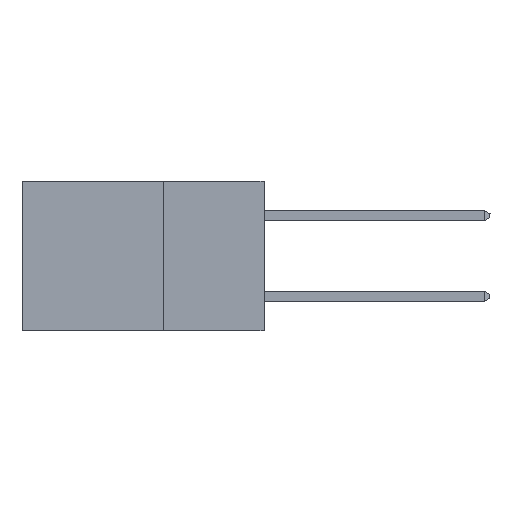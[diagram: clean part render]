
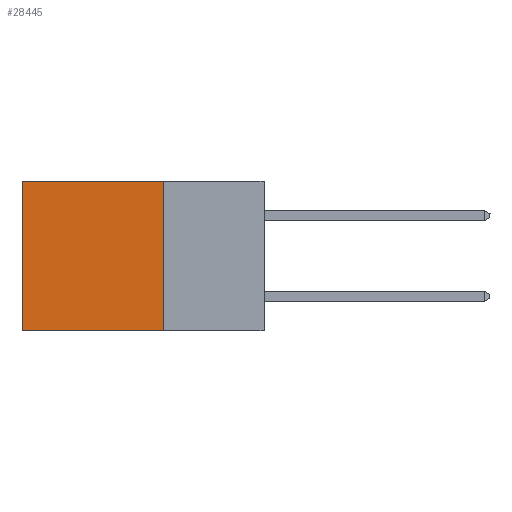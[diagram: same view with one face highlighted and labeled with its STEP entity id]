
A CAD part, left-side view. The second image highlights one B-rep face of the part: STEP entity #28445.
In plain terms, the highlighted planar face has unit normal (-1, 0, 0).
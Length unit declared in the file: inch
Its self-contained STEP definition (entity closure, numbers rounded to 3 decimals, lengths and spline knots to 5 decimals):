
#344 = CARTESIAN_POINT ( 'NONE',  ( 0.298, 0.25, 0. ) ) ;
#1345 = VECTOR ( 'NONE', #23829, 39.37008 ) ;
#2827 = VERTEX_POINT ( 'NONE', #8809 ) ;
#2988 = DIRECTION ( 'NONE',  ( 1., 0., 0. ) ) ;
#3143 = VECTOR ( 'NONE', #20028, 39.37008 ) ;
#3658 = VERTEX_POINT ( 'NONE', #9227 ) ;
#6798 = VERTEX_POINT ( 'NONE', #23408 ) ;
#7547 = CARTESIAN_POINT ( 'NONE',  ( 0.298, 0.6, 0. ) ) ;
#8032 = AXIS2_PLACEMENT_3D ( 'NONE', #344, #2988, #21683 ) ;
#8446 = LINE ( 'NONE', #31696, #1345 ) ;
#8771 = EDGE_CURVE ( 'NONE', #6798, #2827, #8446, .T. ) ;
#8809 = CARTESIAN_POINT ( 'NONE',  ( 0.298, 0.6, 0. ) ) ;
#9227 = CARTESIAN_POINT ( 'NONE',  ( 0.298, 0.6, -0.37 ) ) ;
#9968 = CARTESIAN_POINT ( 'NONE',  ( 0.298, 0.25, 0. ) ) ;
#10212 = LINE ( 'NONE', #7547, #23521 ) ;
#11543 = CARTESIAN_POINT ( 'NONE',  ( 0.298, 0.25, -0.37 ) ) ;
#12288 = ORIENTED_EDGE ( 'NONE', *, *, #25551, .F. ) ;
#12956 = ORIENTED_EDGE ( 'NONE', *, *, #8771, .T. ) ;
#14455 = EDGE_LOOP ( 'NONE', ( #31702, #12288, #31836, #12956 ) ) ;
#16354 = PLANE ( 'NONE',  #8032 ) ;
#17298 = EDGE_CURVE ( 'NONE', #6798, #32842, #17986, .T. ) ;
#17986 = LINE ( 'NONE', #9968, #19663 ) ;
#19663 = VECTOR ( 'NONE', #28549, 39.37008 ) ;
#20028 = DIRECTION ( 'NONE',  ( 0., 1., 0. ) ) ;
#21683 = DIRECTION ( 'NONE',  ( 0., 0., -1. ) ) ;
#22695 = CARTESIAN_POINT ( 'NONE',  ( 0.298, 0.25, -0.37 ) ) ;
#23408 = CARTESIAN_POINT ( 'NONE',  ( 0.298, 0.25, 0. ) ) ;
#23521 = VECTOR ( 'NONE', #28836, 39.37008 ) ;
#23829 = DIRECTION ( 'NONE',  ( 0., 1., 0. ) ) ;
#24427 = LINE ( 'NONE', #22695, #3143 ) ;
#25551 = EDGE_CURVE ( 'NONE', #32842, #3658, #24427, .T. ) ;
#27084 = EDGE_CURVE ( 'NONE', #2827, #3658, #10212, .T. ) ;
#28445 = ADVANCED_FACE ( 'NONE', ( #29639 ), #16354, .F. ) ;
#28549 = DIRECTION ( 'NONE',  ( 0., 0., -1. ) ) ;
#28836 = DIRECTION ( 'NONE',  ( 0., 0., -1. ) ) ;
#29639 = FACE_OUTER_BOUND ( 'NONE', #14455, .T. ) ;
#31696 = CARTESIAN_POINT ( 'NONE',  ( 0.298, 0.25, 0. ) ) ;
#31702 = ORIENTED_EDGE ( 'NONE', *, *, #27084, .T. ) ;
#31836 = ORIENTED_EDGE ( 'NONE', *, *, #17298, .F. ) ;
#32842 = VERTEX_POINT ( 'NONE', #11543 ) ;
